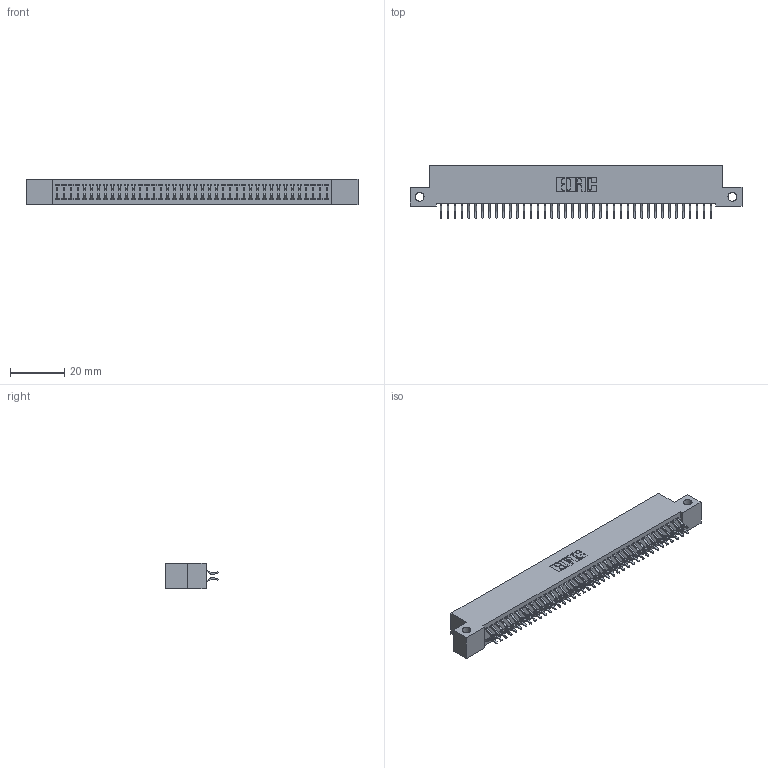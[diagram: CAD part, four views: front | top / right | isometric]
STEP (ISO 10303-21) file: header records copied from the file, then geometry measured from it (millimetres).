
FILE_DESCRIPTION (( 'STEP AP203' ), '1' );
FILE_NAME ('342-080-556-212.STEP', '2019-10-04T11:49:37', ( '' ), ( '' ), 'SwSTEP 2.0', 'SolidWorks 2016', '' );
FILE_SCHEMA (( 'CONFIG_CONTROL_DESIGN' ));
Length unit declared in the file: inch
Products named in the file (3): 342 Part_Side Mount; 345-292-001_556 Tail; 342-080-556-212
Assembly tree (81 placements, depth 2):
  342-080-556-212
    342 Part_Side Mount
    345-292-001_556 Tail  x80
Bounding box: 121.92 x 19.58 x 9.4 mm (x, y, z)
Volume: 10869.1 mm3; surface area: 17405.5 mm2
Topology: 81 solids, 81 shells, 4750 faces, 14139 edges, 9318 vertices
Faces by surface type: plane 3266, cylinder 1484
Entity records: 26083 total; most frequent: CARTESIAN_POINT 4338, ORIENTED_EDGE 4262, DIRECTION 3699, EDGE_CURVE 2131, VECTOR 1995, LINE 1995, VERTEX_POINT 1418, AXIS2_PLACEMENT_3D 852
